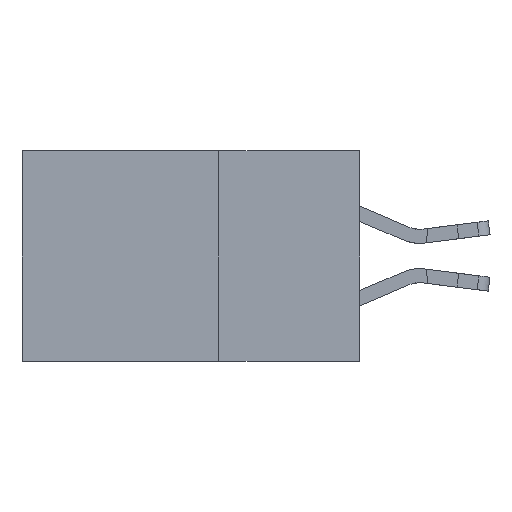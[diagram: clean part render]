
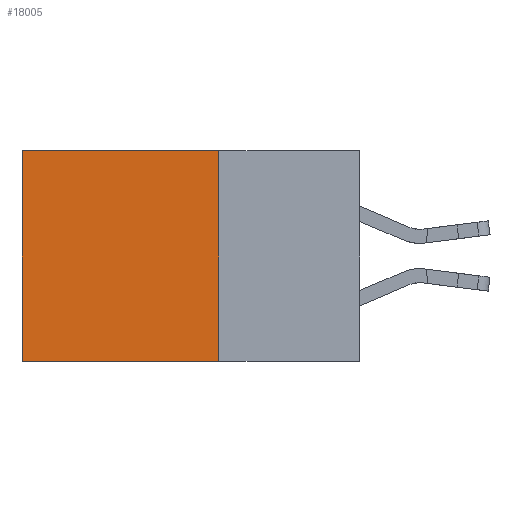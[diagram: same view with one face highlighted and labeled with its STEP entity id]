
A CAD part, left-side view. The second image highlights one B-rep face of the part: STEP entity #18005.
In plain terms, the highlighted planar face has unit normal (-1, 0, 0).
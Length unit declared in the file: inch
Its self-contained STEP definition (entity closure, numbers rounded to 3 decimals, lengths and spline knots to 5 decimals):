
#328 = EDGE_CURVE ( 'NONE', #10481, #7146, #3642, .T. ) ;
#381 = DIRECTION ( 'NONE',  ( 0., 1., 0. ) ) ;
#531 = EDGE_LOOP ( 'NONE', ( #13691, #14058, #12652, #2226 ) ) ;
#678 = LINE ( 'NONE', #18099, #3670 ) ;
#1098 = VECTOR ( 'NONE', #15839, 39.37008 ) ;
#1283 = LINE ( 'NONE', #18812, #5194 ) ;
#1342 = EDGE_CURVE ( 'NONE', #10659, #10481, #8453, .T. ) ;
#1363 = FACE_OUTER_BOUND ( 'NONE', #531, .T. ) ;
#2226 = ORIENTED_EDGE ( 'NONE', *, *, #1342, .T. ) ;
#2430 = CARTESIAN_POINT ( 'NONE',  ( 0.2875, 0.25, -0.375 ) ) ;
#2968 = PLANE ( 'NONE',  #18148 ) ;
#3642 = LINE ( 'NONE', #4135, #14964 ) ;
#3670 = VECTOR ( 'NONE', #381, 39.37008 ) ;
#4135 = CARTESIAN_POINT ( 'NONE',  ( 0.2875, 0.6, -0.375 ) ) ;
#4182 = CARTESIAN_POINT ( 'NONE',  ( 0.2875, 0.25, 0. ) ) ;
#4701 = CARTESIAN_POINT ( 'NONE',  ( 0.2875, 0.6, 0. ) ) ;
#5194 = VECTOR ( 'NONE', #12761, 39.37008 ) ;
#5269 = CARTESIAN_POINT ( 'NONE',  ( 0.2875, 0.25, 0. ) ) ;
#7146 = VERTEX_POINT ( 'NONE', #16618 ) ;
#8453 = LINE ( 'NONE', #4182, #1098 ) ;
#8585 = DIRECTION ( 'NONE',  ( 0., 0., -1. ) ) ;
#8907 = DIRECTION ( 'NONE',  ( 1., 0., 0. ) ) ;
#10481 = VERTEX_POINT ( 'NONE', #4701 ) ;
#10659 = VERTEX_POINT ( 'NONE', #5269 ) ;
#11327 = VERTEX_POINT ( 'NONE', #2430 ) ;
#12652 = ORIENTED_EDGE ( 'NONE', *, *, #15451, .F. ) ;
#12761 = DIRECTION ( 'NONE',  ( 0., 0., -1. ) ) ;
#13120 = EDGE_CURVE ( 'NONE', #11327, #7146, #678, .T. ) ;
#13691 = ORIENTED_EDGE ( 'NONE', *, *, #328, .T. ) ;
#14058 = ORIENTED_EDGE ( 'NONE', *, *, #13120, .F. ) ;
#14589 = CARTESIAN_POINT ( 'NONE',  ( 0.2875, 0.25, -0.375 ) ) ;
#14964 = VECTOR ( 'NONE', #8585, 39.37008 ) ;
#15451 = EDGE_CURVE ( 'NONE', #10659, #11327, #1283, .T. ) ;
#15839 = DIRECTION ( 'NONE',  ( 0., 1., 0. ) ) ;
#16225 = DIRECTION ( 'NONE',  ( 0., 0., -1. ) ) ;
#16618 = CARTESIAN_POINT ( 'NONE',  ( 0.2875, 0.6, -0.375 ) ) ;
#18005 = ADVANCED_FACE ( 'NONE', ( #1363 ), #2968, .F. ) ;
#18099 = CARTESIAN_POINT ( 'NONE',  ( 0.2875, 0.25, -0.375 ) ) ;
#18148 = AXIS2_PLACEMENT_3D ( 'NONE', #14589, #8907, #16225 ) ;
#18812 = CARTESIAN_POINT ( 'NONE',  ( 0.2875, 0.25, -0.375 ) ) ;
